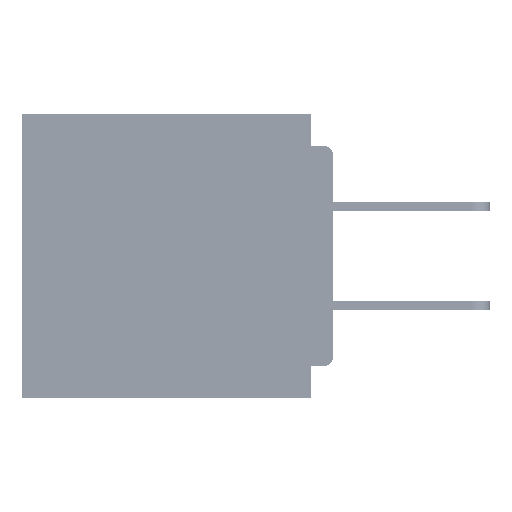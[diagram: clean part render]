
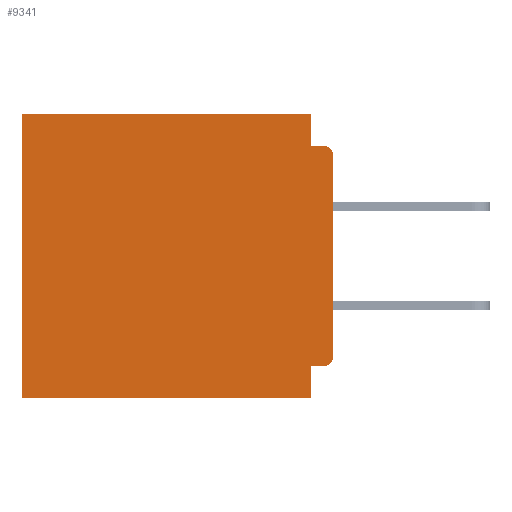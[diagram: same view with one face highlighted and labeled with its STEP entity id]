
A CAD part, left-side view. The second image highlights one B-rep face of the part: STEP entity #9341.
In plain terms, the highlighted planar face has unit normal (-1, 0, 0).
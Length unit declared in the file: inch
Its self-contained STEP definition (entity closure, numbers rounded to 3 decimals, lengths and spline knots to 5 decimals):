
#678 = DIRECTION ( 'NONE',  ( 0., 0., -1. ) ) ;
#1076 = VERTEX_POINT ( 'NONE', #40737 ) ;
#1225 = VERTEX_POINT ( 'NONE', #18317 ) ;
#1266 = EDGE_CURVE ( 'NONE', #18667, #38814, #38439, .T. ) ;
#1648 = CARTESIAN_POINT ( 'NONE',  ( 0.3, 0., -0.4 ) ) ;
#1885 = DIRECTION ( 'NONE',  ( 0., 1., 0. ) ) ;
#1953 = ORIENTED_EDGE ( 'NONE', *, *, #35281, .F. ) ;
#2127 = AXIS2_PLACEMENT_3D ( 'NONE', #13554, #51352, #18976 ) ;
#3270 = DIRECTION ( 'NONE',  ( 0., 1., 0. ) ) ;
#3322 = LINE ( 'NONE', #11427, #16050 ) ;
#4003 = VERTEX_POINT ( 'NONE', #8613 ) ;
#4804 = ORIENTED_EDGE ( 'NONE', *, *, #8876, .T. ) ;
#5669 = CIRCLE ( 'NONE', #2127, 0.015 ) ;
#6141 = DIRECTION ( 'NONE',  ( 0., 0., -1. ) ) ;
#8613 = CARTESIAN_POINT ( 'NONE',  ( 0.3, 0.031, -0.355 ) ) ;
#8876 = EDGE_CURVE ( 'NONE', #67998, #1225, #48010, .T. ) ;
#9341 = ADVANCED_FACE ( 'NONE', ( #31878 ), #63318, .F. ) ;
#11264 = CARTESIAN_POINT ( 'NONE',  ( 0.3, 0.015, -0.34 ) ) ;
#11427 = CARTESIAN_POINT ( 'NONE',  ( 0.3, 0.437, -0.4 ) ) ;
#11553 = ORIENTED_EDGE ( 'NONE', *, *, #21511, .F. ) ;
#12001 = VECTOR ( 'NONE', #64758, 39.37008 ) ;
#12271 = ORIENTED_EDGE ( 'NONE', *, *, #25697, .T. ) ;
#13554 = CARTESIAN_POINT ( 'NONE',  ( 0.3, 0.015, -0.06 ) ) ;
#13779 = EDGE_CURVE ( 'NONE', #64484, #1076, #3322, .T. ) ;
#14120 = LINE ( 'NONE', #56743, #26800 ) ;
#14736 = LINE ( 'NONE', #44795, #27401 ) ;
#16050 = VECTOR ( 'NONE', #678, 39.37008 ) ;
#16694 = DIRECTION ( 'NONE',  ( 0., 0., -1. ) ) ;
#17811 = DIRECTION ( 'NONE',  ( 0., 0., -1. ) ) ;
#18215 = VERTEX_POINT ( 'NONE', #52831 ) ;
#18317 = CARTESIAN_POINT ( 'NONE',  ( 0.3, 0., -0.34 ) ) ;
#18652 = ORIENTED_EDGE ( 'NONE', *, *, #33711, .F. ) ;
#18667 = VERTEX_POINT ( 'NONE', #51580 ) ;
#18976 = DIRECTION ( 'NONE',  ( 0., 0., -1. ) ) ;
#21511 = EDGE_CURVE ( 'NONE', #67998, #4003, #55058, .T. ) ;
#21886 = ORIENTED_EDGE ( 'NONE', *, *, #38804, .T. ) ;
#22297 = CARTESIAN_POINT ( 'NONE',  ( 0.3, 0.031, 0. ) ) ;
#25697 = EDGE_CURVE ( 'NONE', #63197, #64484, #61956, .T. ) ;
#26800 = VECTOR ( 'NONE', #35374, 39.37008 ) ;
#27076 = CARTESIAN_POINT ( 'NONE',  ( 0.3, 0., -0.355 ) ) ;
#27401 = VECTOR ( 'NONE', #17811, 39.37008 ) ;
#30273 = CARTESIAN_POINT ( 'NONE',  ( 0.3, 0., 0. ) ) ;
#31878 = FACE_OUTER_BOUND ( 'NONE', #57732, .T. ) ;
#31917 = CARTESIAN_POINT ( 'NONE',  ( 0.3, 0.015, -0.355 ) ) ;
#32514 = ORIENTED_EDGE ( 'NONE', *, *, #57080, .F. ) ;
#33354 = VECTOR ( 'NONE', #3270, 39.37008 ) ;
#33711 = EDGE_CURVE ( 'NONE', #63197, #18667, #14120, .T. ) ;
#35091 = CARTESIAN_POINT ( 'NONE',  ( 0.3, 0.015, -0.045 ) ) ;
#35281 = EDGE_CURVE ( 'NONE', #4003, #18215, #14736, .T. ) ;
#35374 = DIRECTION ( 'NONE',  ( 0., 0., -1. ) ) ;
#36544 = DIRECTION ( 'NONE',  ( 0., 0., -1. ) ) ;
#37825 = VECTOR ( 'NONE', #6141, 39.37008 ) ;
#38439 = LINE ( 'NONE', #43988, #65332 ) ;
#38593 = CARTESIAN_POINT ( 'NONE',  ( 0.3, 0., -0.4 ) ) ;
#38804 = EDGE_CURVE ( 'NONE', #63655, #38814, #5669, .T. ) ;
#38814 = VERTEX_POINT ( 'NONE', #35091 ) ;
#39195 = EDGE_CURVE ( 'NONE', #63655, #1225, #66366, .T. ) ;
#40737 = CARTESIAN_POINT ( 'NONE',  ( 0.3, 0.437, -0.4 ) ) ;
#40989 = DIRECTION ( 'NONE',  ( 0., -1., 0. ) ) ;
#42575 = ORIENTED_EDGE ( 'NONE', *, *, #13779, .T. ) ;
#43988 = CARTESIAN_POINT ( 'NONE',  ( 0.3, 0., -0.045 ) ) ;
#44195 = AXIS2_PLACEMENT_3D ( 'NONE', #11264, #49088, #16694 ) ;
#44795 = CARTESIAN_POINT ( 'NONE',  ( 0.3, 0.031, -0.4 ) ) ;
#45684 = ORIENTED_EDGE ( 'NONE', *, *, #39195, .F. ) ;
#48010 = CIRCLE ( 'NONE', #44195, 0.015 ) ;
#49088 = DIRECTION ( 'NONE',  ( -1., 0., 0. ) ) ;
#51033 = VECTOR ( 'NONE', #1885, 39.37008 ) ;
#51352 = DIRECTION ( 'NONE',  ( -1., 0., 0. ) ) ;
#51580 = CARTESIAN_POINT ( 'NONE',  ( 0.3, 0.031, -0.045 ) ) ;
#52831 = CARTESIAN_POINT ( 'NONE',  ( 0.3, 0.031, -0.4 ) ) ;
#55058 = LINE ( 'NONE', #27076, #12001 ) ;
#56743 = CARTESIAN_POINT ( 'NONE',  ( 0.3, 0.031, 0. ) ) ;
#57080 = EDGE_CURVE ( 'NONE', #18215, #1076, #65298, .T. ) ;
#57732 = EDGE_LOOP ( 'NONE', ( #45684, #21886, #63996, #18652, #12271, #42575, #32514, #1953, #11553, #4804 ) ) ;
#57938 = CARTESIAN_POINT ( 'NONE',  ( 0.3, 0., -0.4 ) ) ;
#61956 = LINE ( 'NONE', #30273, #33354 ) ;
#63197 = VERTEX_POINT ( 'NONE', #22297 ) ;
#63318 = PLANE ( 'NONE',  #64443 ) ;
#63655 = VERTEX_POINT ( 'NONE', #64215 ) ;
#63996 = ORIENTED_EDGE ( 'NONE', *, *, #1266, .F. ) ;
#64215 = CARTESIAN_POINT ( 'NONE',  ( 0.3, 0., -0.06 ) ) ;
#64443 = AXIS2_PLACEMENT_3D ( 'NONE', #57938, #68688, #36544 ) ;
#64484 = VERTEX_POINT ( 'NONE', #65745 ) ;
#64758 = DIRECTION ( 'NONE',  ( 0., 1., 0. ) ) ;
#65298 = LINE ( 'NONE', #1648, #51033 ) ;
#65332 = VECTOR ( 'NONE', #40989, 39.37008 ) ;
#65745 = CARTESIAN_POINT ( 'NONE',  ( 0.3, 0.437, 0. ) ) ;
#66366 = LINE ( 'NONE', #38593, #37825 ) ;
#67998 = VERTEX_POINT ( 'NONE', #31917 ) ;
#68688 = DIRECTION ( 'NONE',  ( 1., 0., 0. ) ) ;
